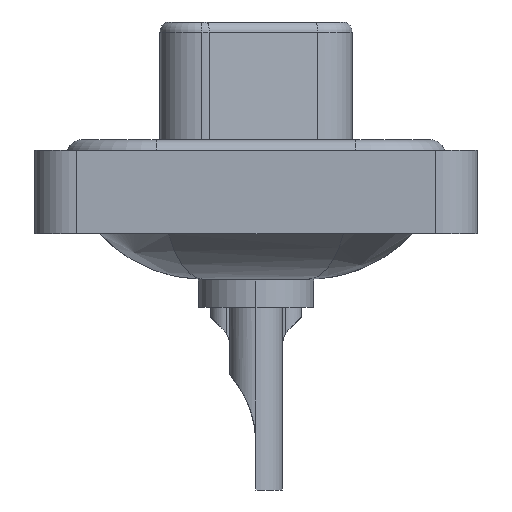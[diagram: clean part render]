
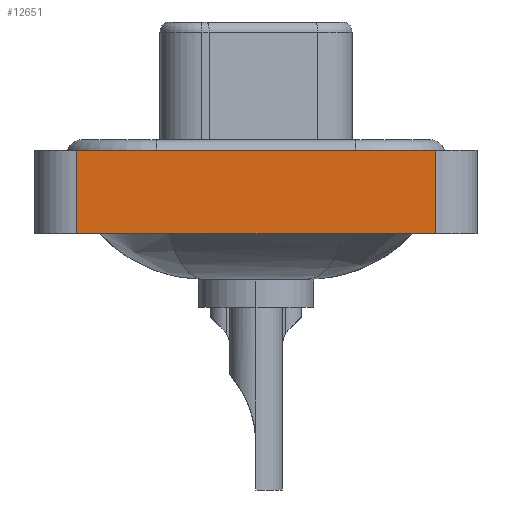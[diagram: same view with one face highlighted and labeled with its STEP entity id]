
A CAD part, left-side view. The second image highlights one B-rep face of the part: STEP entity #12651.
In plain terms, the highlighted planar face has unit normal (-1, 0, 0).
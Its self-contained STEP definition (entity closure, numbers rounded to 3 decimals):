
#409 = VECTOR ( 'NONE', #2725, 1000. ) ;
#581 = VECTOR ( 'NONE', #8944, 1000. ) ;
#1113 = LINE ( 'NONE', #11655, #581 ) ;
#2111 = CARTESIAN_POINT ( 'NONE',  ( -7.3, -8.55, -3.6 ) ) ;
#2725 = DIRECTION ( 'NONE',  ( 0., 0., 1. ) ) ;
#3004 = CARTESIAN_POINT ( 'NONE',  ( -7.3, -8.55, 0.4 ) ) ;
#3098 = CARTESIAN_POINT ( 'NONE',  ( -7.3, -8.55, 0.4 ) ) ;
#3302 = ORIENTED_EDGE ( 'NONE', *, *, #10420, .T. ) ;
#3836 = LINE ( 'NONE', #9426, #18749 ) ;
#3842 = EDGE_LOOP ( 'NONE', ( #3302, #18205, #18105, #17868 ) ) ;
#4102 = CARTESIAN_POINT ( 'NONE',  ( -7.3, 8.55, 0.4 ) ) ;
#4417 = VERTEX_POINT ( 'NONE', #4102 ) ;
#5279 = CARTESIAN_POINT ( 'NONE',  ( -7.3, -8.55, -3.6 ) ) ;
#7037 = VECTOR ( 'NONE', #9974, 1000. ) ;
#7509 = AXIS2_PLACEMENT_3D ( 'NONE', #19547, #11668, #14721 ) ;
#8853 = FACE_OUTER_BOUND ( 'NONE', #3842, .T. ) ;
#8944 = DIRECTION ( 'NONE',  ( 0., 0., 1. ) ) ;
#9038 = CARTESIAN_POINT ( 'NONE',  ( -7.3, 8.55, -3.6 ) ) ;
#9335 = VERTEX_POINT ( 'NONE', #3098 ) ;
#9426 = CARTESIAN_POINT ( 'NONE',  ( -7.3, -8.55, -3.6 ) ) ;
#9974 = DIRECTION ( 'NONE',  ( 0., -1., 0. ) ) ;
#10359 = PLANE ( 'NONE',  #7509 ) ;
#10420 = EDGE_CURVE ( 'NONE', #14267, #9335, #14793, .T. ) ;
#10529 = LINE ( 'NONE', #3004, #7037 ) ;
#11655 = CARTESIAN_POINT ( 'NONE',  ( -7.3, 8.55, -3.6 ) ) ;
#11668 = DIRECTION ( 'NONE',  ( -1., 0., 0. ) ) ;
#12651 = ADVANCED_FACE ( 'NONE', ( #8853 ), #10359, .T. ) ;
#12874 = DIRECTION ( 'NONE',  ( 0., -1., 0. ) ) ;
#13185 = VERTEX_POINT ( 'NONE', #9038 ) ;
#14267 = VERTEX_POINT ( 'NONE', #2111 ) ;
#14400 = EDGE_CURVE ( 'NONE', #13185, #4417, #1113, .T. ) ;
#14721 = DIRECTION ( 'NONE',  ( 0., 0., 1. ) ) ;
#14793 = LINE ( 'NONE', #5279, #409 ) ;
#16162 = EDGE_CURVE ( 'NONE', #4417, #9335, #10529, .T. ) ;
#17868 = ORIENTED_EDGE ( 'NONE', *, *, #18278, .T. ) ;
#18105 = ORIENTED_EDGE ( 'NONE', *, *, #14400, .F. ) ;
#18205 = ORIENTED_EDGE ( 'NONE', *, *, #16162, .F. ) ;
#18278 = EDGE_CURVE ( 'NONE', #13185, #14267, #3836, .T. ) ;
#18749 = VECTOR ( 'NONE', #12874, 1000. ) ;
#19547 = CARTESIAN_POINT ( 'NONE',  ( -7.3, -8.55, -3.6 ) ) ;
